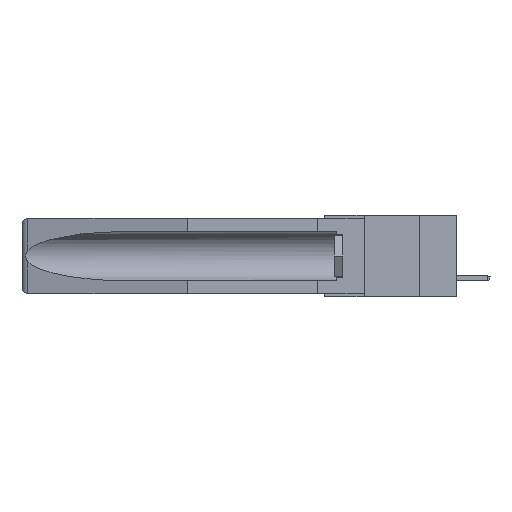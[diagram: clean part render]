
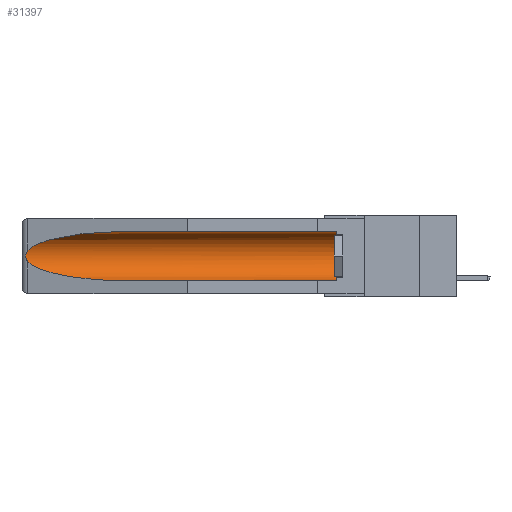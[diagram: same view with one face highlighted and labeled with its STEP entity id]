
A CAD part, left-side view. The second image highlights one B-rep face of the part: STEP entity #31397.
In plain terms, the highlighted cylindrical face has radius 2.857 mm (diameter 5.715 mm), a partial arc.
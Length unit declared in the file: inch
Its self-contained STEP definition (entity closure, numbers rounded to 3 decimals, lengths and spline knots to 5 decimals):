
#519 = VECTOR ( 'NONE', #5680, 39.37008 ) ;
#617 = VECTOR ( 'NONE', #27198, 39.37008 ) ;
#844 = ORIENTED_EDGE ( 'NONE', *, *, #30024, .F. ) ;
#1094 = B_SPLINE_CURVE_WITH_KNOTS ( 'NONE', 3,
 ( #3533, #6114, #3652, #29261, #31868, #21601, #24144, #3875, #1379, #32083 ),
 .UNSPECIFIED., .F., .F.,
 ( 4, 2, 2, 2, 4 ),
 ( 0., 0.00029, 0.00058, 0.00087, 0.00117 ),
 .UNSPECIFIED. ) ;
#1179 = VERTEX_POINT ( 'NONE', #5186 ) ;
#1379 = CARTESIAN_POINT ( 'NONE',  ( 0.26597, 1.5296, -0.19026 ) ) ;
#3023 = CARTESIAN_POINT ( 'NONE',  ( 0.155, -0.30754, -0.1715 ) ) ;
#3533 = CARTESIAN_POINT ( 'NONE',  ( 0.26537, 1.52718, -0.14972 ) ) ;
#3625 = ORIENTED_EDGE ( 'NONE', *, *, #26151, .T. ) ;
#3652 = CARTESIAN_POINT ( 'NONE',  ( 0.26654, 1.53092, -0.15636 ) ) ;
#3875 = CARTESIAN_POINT ( 'NONE',  ( 0.26655, 1.53094, -0.18657 ) ) ;
#4545 = ORIENTED_EDGE ( 'NONE', *, *, #13377, .T. ) ;
#4938 = LINE ( 'NONE', #20939, #519 ) ;
#5186 = CARTESIAN_POINT ( 'NONE',  ( 0.155, 0.126, -0.059 ) ) ;
#5680 = DIRECTION ( 'NONE',  ( 0., 1., 0. ) ) ;
#5843 = DIRECTION ( 'NONE',  ( 0., 1., 0. ) ) ;
#6114 = CARTESIAN_POINT ( 'NONE',  ( 0.26597, 1.52961, -0.15275 ) ) ;
#6364 = AXIS2_PLACEMENT_3D ( 'NONE', #16885, #6782, #29359 ) ;
#6782 = DIRECTION ( 'NONE',  ( 0., -1., 0. ) ) ;
#6802 = CARTESIAN_POINT ( 'NONE',  ( 0.26537, 1.52718, -0.19328 ) ) ;
#7177 = EDGE_CURVE ( 'NONE', #26706, #1179, #14990, .T. ) ;
#7794 = CARTESIAN_POINT ( 'NONE',  ( 0.155, 1.07973, -0.059 ) ) ;
#7936 = VERTEX_POINT ( 'NONE', #27105 ) ;
#8123 = CARTESIAN_POINT ( 'NONE',  ( 0.26537, 1.52718, -0.14972 ) ) ;
#8389 = DIRECTION ( 'NONE',  ( 0., 0., 1. ) ) ;
#8774 = CARTESIAN_POINT ( 'NONE',  ( 0.26537, 1.52718, -0.19328 ) ) ;
#10262 = CYLINDRICAL_SURFACE ( 'NONE', #26096, 0.1125 ) ;
#10595 = CARTESIAN_POINT ( 'NONE',  ( 0.25451, 1.48313, -0.09465 ) ) ;
#11201 = VERTEX_POINT ( 'NONE', #6802 ) ;
#11630 = CARTESIAN_POINT ( 'NONE',  ( 0.155, -0.30754, -0.059 ) ) ;
#13377 = EDGE_CURVE ( 'NONE', #11201, #7936, #22910, .T. ) ;
#14318 = EDGE_CURVE ( 'NONE', #1179, #26135, #20705, .T. ) ;
#14990 = CIRCLE ( 'NONE', #6364, 0.1125 ) ;
#16885 = CARTESIAN_POINT ( 'NONE',  ( 0.155, 0.126, -0.1715 ) ) ;
#18039 = CARTESIAN_POINT ( 'NONE',  ( 0.155, 1.07973, -0.059 ) ) ;
#19262 = CARTESIAN_POINT ( 'NONE',  ( 0.155, 1.07973, -0.284 ) ) ;
#19278 = CARTESIAN_POINT ( 'NONE',  ( 0.26537, 1.52718, -0.14972 ) ) ;
#20705 = LINE ( 'NONE', #11630, #617 ) ;
#20733 = CARTESIAN_POINT ( 'NONE',  ( 0.21114, 1.30732, -0.059 ) ) ;
#20939 = CARTESIAN_POINT ( 'NONE',  ( 0.155, -0.30754, -0.284 ) ) ;
#21601 = CARTESIAN_POINT ( 'NONE',  ( 0.2675, 1.53308, -0.17534 ) ) ;
#21629 = EDGE_LOOP ( 'NONE', ( #3625, #30141, #4545, #844, #24031, #31810 ) ) ;
#22367 = VERTEX_POINT ( 'NONE', #19278 ) ;
#22910 =( BOUNDED_CURVE ( )  B_SPLINE_CURVE ( 3, ( #8774, #26593, #26711, #19262 ),
 .UNSPECIFIED., .F., .F. ) 
 B_SPLINE_CURVE_WITH_KNOTS ( ( 4, 4 ),
 ( 0.1948, 1.5708 ),
 .UNSPECIFIED. ) 
 CURVE ( )  GEOMETRIC_REPRESENTATION_ITEM ( )  RATIONAL_B_SPLINE_CURVE ( ( 1., 0.848, 0.848, 1. ) ) 
 REPRESENTATION_ITEM ( '' )  );
#24031 = ORIENTED_EDGE ( 'NONE', *, *, #7177, .T. ) ;
#24144 = CARTESIAN_POINT ( 'NONE',  ( 0.2673, 1.53269, -0.17917 ) ) ;
#25958 =( BOUNDED_CURVE ( )  B_SPLINE_CURVE ( 3, ( #7794, #20733, #10595, #8123 ),
 .UNSPECIFIED., .F., .F. ) 
 B_SPLINE_CURVE_WITH_KNOTS ( ( 4, 4 ),
 ( 4.71239, 6.08839 ),
 .UNSPECIFIED. ) 
 CURVE ( )  GEOMETRIC_REPRESENTATION_ITEM ( )  RATIONAL_B_SPLINE_CURVE ( ( 1., 0.848, 0.848, 1. ) ) 
 REPRESENTATION_ITEM ( '' )  );
#26096 = AXIS2_PLACEMENT_3D ( 'NONE', #3023, #5843, #8389 ) ;
#26135 = VERTEX_POINT ( 'NONE', #18039 ) ;
#26151 = EDGE_CURVE ( 'NONE', #26135, #22367, #25958, .T. ) ;
#26593 = CARTESIAN_POINT ( 'NONE',  ( 0.25451, 1.48313, -0.24835 ) ) ;
#26706 = VERTEX_POINT ( 'NONE', #31989 ) ;
#26711 = CARTESIAN_POINT ( 'NONE',  ( 0.21114, 1.30732, -0.284 ) ) ;
#27105 = CARTESIAN_POINT ( 'NONE',  ( 0.155, 1.07973, -0.284 ) ) ;
#27198 = DIRECTION ( 'NONE',  ( 0., 1., 0. ) ) ;
#29261 = CARTESIAN_POINT ( 'NONE',  ( 0.2673, 1.5327, -0.16383 ) ) ;
#29359 = DIRECTION ( 'NONE',  ( 0., 0., 1. ) ) ;
#30024 = EDGE_CURVE ( 'NONE', #26706, #7936, #4938, .T. ) ;
#30141 = ORIENTED_EDGE ( 'NONE', *, *, #30217, .T. ) ;
#30217 = EDGE_CURVE ( 'NONE', #22367, #11201, #1094, .T. ) ;
#31397 = ADVANCED_FACE ( 'NONE', ( #32321 ), #10262, .F. ) ;
#31810 = ORIENTED_EDGE ( 'NONE', *, *, #14318, .T. ) ;
#31868 = CARTESIAN_POINT ( 'NONE',  ( 0.2675, 1.53308, -0.16763 ) ) ;
#31989 = CARTESIAN_POINT ( 'NONE',  ( 0.155, 0.126, -0.284 ) ) ;
#32083 = CARTESIAN_POINT ( 'NONE',  ( 0.26537, 1.52718, -0.19328 ) ) ;
#32321 = FACE_OUTER_BOUND ( 'NONE', #21629, .T. ) ;
